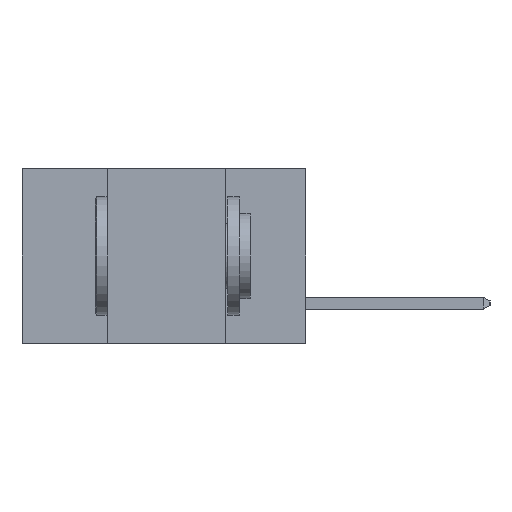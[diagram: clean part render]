
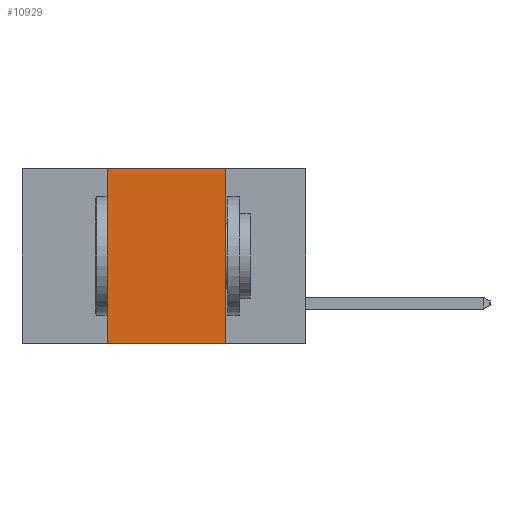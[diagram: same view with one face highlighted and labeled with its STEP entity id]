
A CAD part, left-side view. The second image highlights one B-rep face of the part: STEP entity #10929.
In plain terms, the highlighted planar face has unit normal (-1, 0, 0).
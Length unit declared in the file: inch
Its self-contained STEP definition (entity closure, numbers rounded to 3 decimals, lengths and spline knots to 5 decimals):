
#143 = CARTESIAN_POINT ( 'NONE',  ( 0., 0.6, 0. ) ) ;
#206 = EDGE_CURVE ( 'NONE', #1929, #10198, #6400, .T. ) ;
#1156 = ORIENTED_EDGE ( 'NONE', *, *, #206, .F. ) ;
#1571 = DIRECTION ( 'NONE',  ( 0., -1., 0. ) ) ;
#1605 = CARTESIAN_POINT ( 'NONE',  ( 0., 0.6, -0.37 ) ) ;
#1929 = VERTEX_POINT ( 'NONE', #21691 ) ;
#2016 = LINE ( 'NONE', #1605, #16322 ) ;
#2114 = DIRECTION ( 'NONE',  ( 1., 0., 0. ) ) ;
#2118 = FACE_OUTER_BOUND ( 'NONE', #11775, .T. ) ;
#3586 = CARTESIAN_POINT ( 'NONE',  ( 0., 0.42, 0. ) ) ;
#4016 = VECTOR ( 'NONE', #19481, 39.37008 ) ;
#4057 = AXIS2_PLACEMENT_3D ( 'NONE', #143, #2114, #16343 ) ;
#5697 = CARTESIAN_POINT ( 'NONE',  ( 0., 0.17, -0.37 ) ) ;
#6400 = LINE ( 'NONE', #17592, #13098 ) ;
#6420 = VERTEX_POINT ( 'NONE', #7371 ) ;
#6602 = EDGE_CURVE ( 'NONE', #1929, #20311, #2016, .T. ) ;
#7371 = CARTESIAN_POINT ( 'NONE',  ( 0., 0.17, 0. ) ) ;
#9717 = ORIENTED_EDGE ( 'NONE', *, *, #10474, .F. ) ;
#10198 = VERTEX_POINT ( 'NONE', #3586 ) ;
#10474 = EDGE_CURVE ( 'NONE', #6420, #20311, #13617, .T. ) ;
#10929 = ADVANCED_FACE ( 'NONE', ( #2118 ), #12246, .F. ) ;
#11775 = EDGE_LOOP ( 'NONE', ( #9717, #25096, #1156, #16694 ) ) ;
#12246 = PLANE ( 'NONE',  #4057 ) ;
#12527 = DIRECTION ( 'NONE',  ( 0., 0., -1. ) ) ;
#13098 = VECTOR ( 'NONE', #17661, 39.37008 ) ;
#13617 = LINE ( 'NONE', #20622, #14245 ) ;
#14245 = VECTOR ( 'NONE', #12527, 39.37008 ) ;
#14801 = LINE ( 'NONE', #17465, #4016 ) ;
#16322 = VECTOR ( 'NONE', #1571, 39.37008 ) ;
#16343 = DIRECTION ( 'NONE',  ( 0., 0., -1. ) ) ;
#16694 = ORIENTED_EDGE ( 'NONE', *, *, #6602, .T. ) ;
#17465 = CARTESIAN_POINT ( 'NONE',  ( 0., 0.6, 0. ) ) ;
#17592 = CARTESIAN_POINT ( 'NONE',  ( 0., 0.42, -0.37 ) ) ;
#17661 = DIRECTION ( 'NONE',  ( 0., 0., 1. ) ) ;
#19481 = DIRECTION ( 'NONE',  ( 0., -1., 0. ) ) ;
#20311 = VERTEX_POINT ( 'NONE', #5697 ) ;
#20622 = CARTESIAN_POINT ( 'NONE',  ( 0., 0.17, -0.37 ) ) ;
#21691 = CARTESIAN_POINT ( 'NONE',  ( 0., 0.42, -0.37 ) ) ;
#23436 = EDGE_CURVE ( 'NONE', #10198, #6420, #14801, .T. ) ;
#25096 = ORIENTED_EDGE ( 'NONE', *, *, #23436, .F. ) ;
